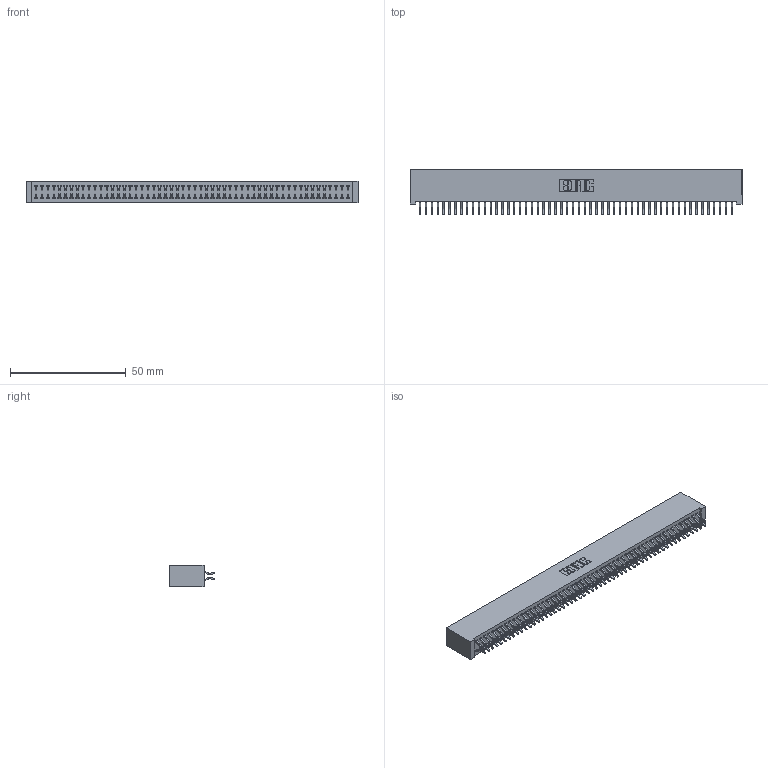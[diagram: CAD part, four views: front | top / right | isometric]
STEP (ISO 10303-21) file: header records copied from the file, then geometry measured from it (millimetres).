
FILE_DESCRIPTION (( 'STEP AP203' ), '1' );
FILE_NAME ('342-108-556-201.STEP', '2019-10-04T19:56:35', ( '' ), ( '' ), 'SwSTEP 2.0', 'SolidWorks 2016', '' );
FILE_SCHEMA (( 'CONFIG_CONTROL_DESIGN' ));
Length unit declared in the file: inch
Products named in the file (3): 342 Part_Lugless; 345-292-001_556 Tail; 342-108-556-201
Assembly tree (109 placements, depth 2):
  342-108-556-201
    342 Part_Lugless
    345-292-001_556 Tail  x108
Bounding box: 143.41 x 19.58 x 9.4 mm (x, y, z)
Volume: 13378.8 mm3; surface area: 22414.5 mm2
Topology: 109 solids, 109 shells, 6366 faces, 18959 edges, 12494 vertices
Faces by surface type: plane 4382, cylinder 1984
Entity records: 32999 total; most frequent: CARTESIAN_POINT 5466, ORIENTED_EDGE 5390, DIRECTION 4631, EDGE_CURVE 2695, LINE 2567, VECTOR 2567, VERTEX_POINT 1794, AXIS2_PLACEMENT_3D 1032
